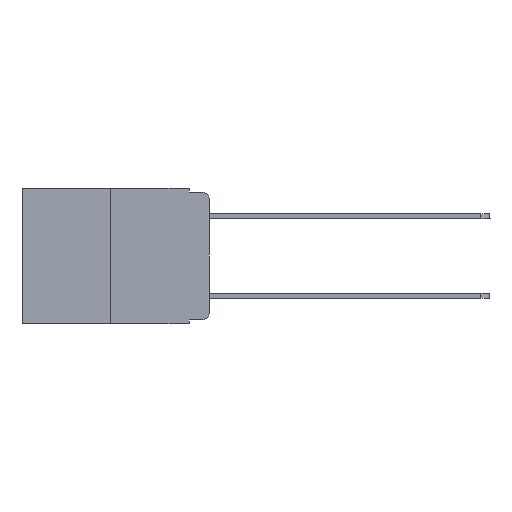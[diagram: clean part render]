
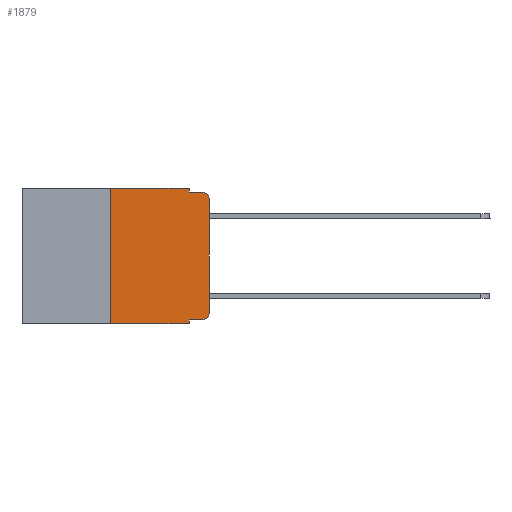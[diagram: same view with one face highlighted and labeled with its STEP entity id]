
A CAD part, left-side view. The second image highlights one B-rep face of the part: STEP entity #1879.
In plain terms, the highlighted planar face has unit normal (-1, 0, 0).
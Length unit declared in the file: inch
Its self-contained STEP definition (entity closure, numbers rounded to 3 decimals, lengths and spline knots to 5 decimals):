
#145 = EDGE_CURVE ( 'NONE', #5799, #13541, #3476, .T. ) ;
#185 = CARTESIAN_POINT ( 'NONE',  ( 0., 0.02, -0.333 ) ) ;
#206 = CARTESIAN_POINT ( 'NONE',  ( 0., 0.25, -0.343 ) ) ;
#306 = ORIENTED_EDGE ( 'NONE', *, *, #19758, .F. ) ;
#317 = ORIENTED_EDGE ( 'NONE', *, *, #19518, .T. ) ;
#392 = DIRECTION ( 'NONE',  ( 0., 0., -1. ) ) ;
#416 = ORIENTED_EDGE ( 'NONE', *, *, #15846, .F. ) ;
#745 = CARTESIAN_POINT ( 'NONE',  ( 0., 0.25, 0. ) ) ;
#859 = ORIENTED_EDGE ( 'NONE', *, *, #18908, .F. ) ;
#1356 = CARTESIAN_POINT ( 'NONE',  ( 0., 0., 0. ) ) ;
#1482 = CARTESIAN_POINT ( 'NONE',  ( 0., 0.25, 0. ) ) ;
#1879 = ADVANCED_FACE ( 'NONE', ( #2890 ), #12165, .F. ) ;
#2890 = FACE_OUTER_BOUND ( 'NONE', #20322, .T. ) ;
#2914 = DIRECTION ( 'NONE',  ( 0., 0., -1. ) ) ;
#3283 = VERTEX_POINT ( 'NONE', #19494 ) ;
#3363 = VECTOR ( 'NONE', #16528, 39.37008 ) ;
#3476 = LINE ( 'NONE', #20110, #15906 ) ;
#3523 = VERTEX_POINT ( 'NONE', #745 ) ;
#3769 = CARTESIAN_POINT ( 'NONE',  ( 0., 0.051, -0.01 ) ) ;
#4083 = EDGE_CURVE ( 'NONE', #13541, #3283, #4656, .T. ) ;
#4656 = CIRCLE ( 'NONE', #20546, 0.02 ) ;
#4662 = LINE ( 'NONE', #21629, #8894 ) ;
#4859 = VECTOR ( 'NONE', #16508, 39.37008 ) ;
#5376 = EDGE_CURVE ( 'NONE', #11982, #3523, #17037, .T. ) ;
#5799 = VERTEX_POINT ( 'NONE', #6093 ) ;
#6093 = CARTESIAN_POINT ( 'NONE',  ( 0., 0.051, -0.333 ) ) ;
#6228 = DIRECTION ( 'NONE',  ( 0., -1., 0. ) ) ;
#6413 = DIRECTION ( 'NONE',  ( 0., -1., 0. ) ) ;
#6434 = DIRECTION ( 'NONE',  ( -1., 0., 0. ) ) ;
#6760 = VERTEX_POINT ( 'NONE', #13107 ) ;
#7025 = ORIENTED_EDGE ( 'NONE', *, *, #9338, .T. ) ;
#7332 = LINE ( 'NONE', #11345, #7606 ) ;
#7606 = VECTOR ( 'NONE', #2914, 39.37008 ) ;
#7826 = CARTESIAN_POINT ( 'NONE',  ( 0., 0.051, -0.01 ) ) ;
#8500 = VERTEX_POINT ( 'NONE', #7826 ) ;
#8894 = VECTOR ( 'NONE', #6413, 39.37008 ) ;
#9106 = AXIS2_PLACEMENT_3D ( 'NONE', #12024, #15403, #392 ) ;
#9338 = EDGE_CURVE ( 'NONE', #3283, #16235, #11562, .T. ) ;
#9687 = EDGE_CURVE ( 'NONE', #11982, #9928, #4662, .T. ) ;
#9928 = VERTEX_POINT ( 'NONE', #10591 ) ;
#10041 = ORIENTED_EDGE ( 'NONE', *, *, #4083, .T. ) ;
#10591 = CARTESIAN_POINT ( 'NONE',  ( 0., 0.051, -0.343 ) ) ;
#10886 = ORIENTED_EDGE ( 'NONE', *, *, #20651, .F. ) ;
#10976 = CIRCLE ( 'NONE', #19009, 0.02 ) ;
#11176 = VECTOR ( 'NONE', #12133, 39.37008 ) ;
#11345 = CARTESIAN_POINT ( 'NONE',  ( 0., 0.051, 0. ) ) ;
#11562 = LINE ( 'NONE', #1356, #3363 ) ;
#11664 = CARTESIAN_POINT ( 'NONE',  ( 0., 0., -0.03 ) ) ;
#11982 = VERTEX_POINT ( 'NONE', #206 ) ;
#12024 = CARTESIAN_POINT ( 'NONE',  ( 0., 0.473, 0. ) ) ;
#12026 = VECTOR ( 'NONE', #20677, 39.37008 ) ;
#12133 = DIRECTION ( 'NONE',  ( 0., -1., 0. ) ) ;
#12165 = PLANE ( 'NONE',  #9106 ) ;
#12555 = LINE ( 'NONE', #12961, #17857 ) ;
#12961 = CARTESIAN_POINT ( 'NONE',  ( 0., 0.473, 0. ) ) ;
#13042 = ORIENTED_EDGE ( 'NONE', *, *, #145, .T. ) ;
#13107 = CARTESIAN_POINT ( 'NONE',  ( 0., 0.02, -0.01 ) ) ;
#13111 = LINE ( 'NONE', #20750, #12026 ) ;
#13303 = DIRECTION ( 'NONE',  ( 0., 0., -1. ) ) ;
#13541 = VERTEX_POINT ( 'NONE', #185 ) ;
#14655 = DIRECTION ( 'NONE',  ( 0., -1., 0. ) ) ;
#15403 = DIRECTION ( 'NONE',  ( 1., 0., 0. ) ) ;
#15846 = EDGE_CURVE ( 'NONE', #8500, #6760, #20240, .T. ) ;
#15906 = VECTOR ( 'NONE', #6228, 39.37008 ) ;
#16235 = VERTEX_POINT ( 'NONE', #11664 ) ;
#16501 = CARTESIAN_POINT ( 'NONE',  ( 0., 0.02, -0.313 ) ) ;
#16508 = DIRECTION ( 'NONE',  ( 0., 0., 1. ) ) ;
#16528 = DIRECTION ( 'NONE',  ( 0., 0., 1. ) ) ;
#16574 = CARTESIAN_POINT ( 'NONE',  ( 0., 0.02, -0.03 ) ) ;
#17037 = LINE ( 'NONE', #1482, #4859 ) ;
#17857 = VECTOR ( 'NONE', #14655, 39.37008 ) ;
#18268 = DIRECTION ( 'NONE',  ( -1., 0., 0. ) ) ;
#18805 = CARTESIAN_POINT ( 'NONE',  ( 0., 0.051, 0. ) ) ;
#18908 = EDGE_CURVE ( 'NONE', #21721, #8500, #7332, .T. ) ;
#19009 = AXIS2_PLACEMENT_3D ( 'NONE', #16574, #6434, #13303 ) ;
#19273 = ORIENTED_EDGE ( 'NONE', *, *, #5376, .F. ) ;
#19494 = CARTESIAN_POINT ( 'NONE',  ( 0., 0., -0.313 ) ) ;
#19518 = EDGE_CURVE ( 'NONE', #16235, #6760, #10976, .T. ) ;
#19758 = EDGE_CURVE ( 'NONE', #5799, #9928, #13111, .T. ) ;
#19890 = DIRECTION ( 'NONE',  ( 0., 0., -1. ) ) ;
#20110 = CARTESIAN_POINT ( 'NONE',  ( 0., 0.051, -0.333 ) ) ;
#20240 = LINE ( 'NONE', #3769, #11176 ) ;
#20322 = EDGE_LOOP ( 'NONE', ( #7025, #317, #416, #859, #10886, #19273, #21160, #306, #13042, #10041 ) ) ;
#20546 = AXIS2_PLACEMENT_3D ( 'NONE', #16501, #18268, #19890 ) ;
#20651 = EDGE_CURVE ( 'NONE', #3523, #21721, #12555, .T. ) ;
#20677 = DIRECTION ( 'NONE',  ( 0., 0., -1. ) ) ;
#20750 = CARTESIAN_POINT ( 'NONE',  ( 0., 0.051, 0. ) ) ;
#21160 = ORIENTED_EDGE ( 'NONE', *, *, #9687, .T. ) ;
#21629 = CARTESIAN_POINT ( 'NONE',  ( 0., 0.473, -0.343 ) ) ;
#21721 = VERTEX_POINT ( 'NONE', #18805 ) ;
